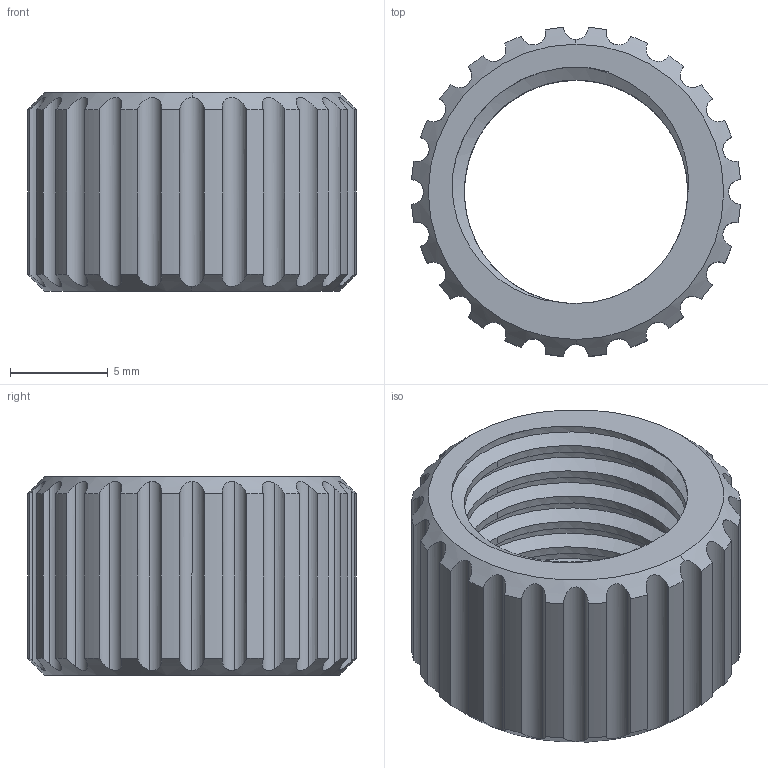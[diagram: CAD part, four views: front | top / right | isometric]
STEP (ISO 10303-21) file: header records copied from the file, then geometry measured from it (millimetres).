
FILE_DESCRIPTION (( 'STEP AP203' ), '1' );
FILE_NAME ('AF-HF-LR-PRT-007-STEP.STEP', '2020-10-30T14:18:35', ( '' ), ( '' ), 'SwSTEP 2.0', 'SolidWorks 2018', '' );
FILE_SCHEMA (( 'CONFIG_CONTROL_DESIGN' ));
Length unit declared in the file: inch
Products named in the file (1): AF-HF-LR-PRT-007-STEP
Bounding box: 16.83 x 16.83 x 10.16 mm (x, y, z)
Volume: 930.5 mm3; surface area: 1404.1 mm2
Topology: 1 solids, 1 shells, 82 faces, 240 edges, 160 vertices
Faces by surface type: cylinder 73, cone 4, bspline 3, plane 2
Entity records: 5124 total; most frequent: CARTESIAN_POINT 3064, ORIENTED_EDGE 480, DIRECTION 346, EDGE_CURVE 240, VERTEX_POINT 160, AXIS2_PLACEMENT_3D 135, EDGE_LOOP 84, FACE_OUTER_BOUND 82
